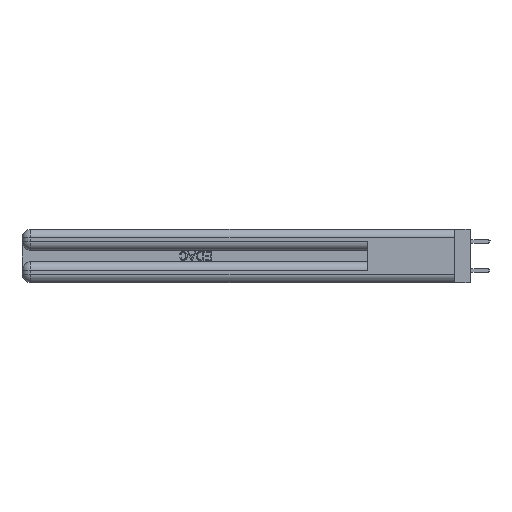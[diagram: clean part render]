
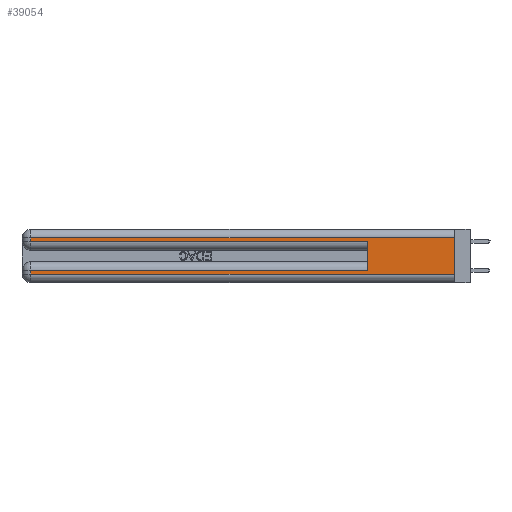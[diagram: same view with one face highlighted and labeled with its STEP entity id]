
A CAD part, left-side view. The second image highlights one B-rep face of the part: STEP entity #39054.
In plain terms, the highlighted planar face has unit normal (-1, 0, 0).
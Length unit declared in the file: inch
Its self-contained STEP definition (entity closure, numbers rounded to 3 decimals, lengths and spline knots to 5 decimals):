
#481 = EDGE_LOOP ( 'NONE', ( #45113, #39682, #36424, #28105, #32733, #26365, #26981, #19928 ) ) ;
#1078 = CARTESIAN_POINT ( 'NONE',  ( 0., 0.6, 0.145 ) ) ;
#2866 = DIRECTION ( 'NONE',  ( 0., 0., -1. ) ) ;
#3239 = CARTESIAN_POINT ( 'NONE',  ( 0., 0.6, 0.085 ) ) ;
#3353 = DIRECTION ( 'NONE',  ( 0., 1., 0. ) ) ;
#3732 = VERTEX_POINT ( 'NONE', #3239 ) ;
#5696 = DIRECTION ( 'NONE',  ( 1., 0., 0. ) ) ;
#6224 = VECTOR ( 'NONE', #2866, 39.37008 ) ;
#7270 = CARTESIAN_POINT ( 'NONE',  ( 0., 0., 0.285 ) ) ;
#7310 = DIRECTION ( 'NONE',  ( 0., 1., 0. ) ) ;
#7464 = LINE ( 'NONE', #50279, #6224 ) ;
#8443 = FACE_OUTER_BOUND ( 'NONE', #481, .T. ) ;
#10803 = LINE ( 'NONE', #7270, #39907 ) ;
#11303 = DIRECTION ( 'NONE',  ( 0., -1., 0. ) ) ;
#11485 = VERTEX_POINT ( 'NONE', #17753 ) ;
#12801 = CARTESIAN_POINT ( 'NONE',  ( 0., 0.6, 0.285 ) ) ;
#16050 = EDGE_CURVE ( 'NONE', #3732, #44000, #24509, .T. ) ;
#16566 = CARTESIAN_POINT ( 'NONE',  ( 0., 2.94, 0.085 ) ) ;
#17489 = VECTOR ( 'NONE', #24978, 39.37008 ) ;
#17753 = CARTESIAN_POINT ( 'NONE',  ( 0., 2.94, 0.06 ) ) ;
#18717 = LINE ( 'NONE', #1078, #17489 ) ;
#19928 = ORIENTED_EDGE ( 'NONE', *, *, #29852, .T. ) ;
#20845 = LINE ( 'NONE', #24901, #50983 ) ;
#24063 = EDGE_CURVE ( 'NONE', #33471, #24924, #10803, .T. ) ;
#24100 = AXIS2_PLACEMENT_3D ( 'NONE', #33316, #5696, #33477 ) ;
#24509 = LINE ( 'NONE', #42962, #33781 ) ;
#24901 = CARTESIAN_POINT ( 'NONE',  ( 0., 2.94, 0.37 ) ) ;
#24924 = VERTEX_POINT ( 'NONE', #12801 ) ;
#24978 = DIRECTION ( 'NONE',  ( 0., 0., 1. ) ) ;
#26365 = ORIENTED_EDGE ( 'NONE', *, *, #16050, .T. ) ;
#26981 = ORIENTED_EDGE ( 'NONE', *, *, #51088, .T. ) ;
#27733 = VECTOR ( 'NONE', #3353, 39.37008 ) ;
#28105 = ORIENTED_EDGE ( 'NONE', *, *, #24063, .T. ) ;
#28912 = DIRECTION ( 'NONE',  ( 0., 0., -1. ) ) ;
#29246 = VECTOR ( 'NONE', #35326, 39.37008 ) ;
#29548 = PLANE ( 'NONE',  #24100 ) ;
#29852 = EDGE_CURVE ( 'NONE', #11485, #31532, #30468, .T. ) ;
#30468 = LINE ( 'NONE', #31371, #29246 ) ;
#31371 = CARTESIAN_POINT ( 'NONE',  ( 0., 0., 0.06 ) ) ;
#31532 = VERTEX_POINT ( 'NONE', #33469 ) ;
#32722 = EDGE_CURVE ( 'NONE', #33329, #31532, #34468, .T. ) ;
#32733 = ORIENTED_EDGE ( 'NONE', *, *, #42719, .F. ) ;
#33246 = VECTOR ( 'NONE', #37517, 39.37008 ) ;
#33316 = CARTESIAN_POINT ( 'NONE',  ( 0., 0., 0.37 ) ) ;
#33329 = VERTEX_POINT ( 'NONE', #40905 ) ;
#33469 = CARTESIAN_POINT ( 'NONE',  ( 0., 0., 0.06 ) ) ;
#33471 = VERTEX_POINT ( 'NONE', #37632 ) ;
#33477 = DIRECTION ( 'NONE',  ( 0., 0., -1. ) ) ;
#33537 = CARTESIAN_POINT ( 'NONE',  ( 0., 0., 0.37 ) ) ;
#33781 = VECTOR ( 'NONE', #7310, 39.37008 ) ;
#34468 = LINE ( 'NONE', #33537, #33246 ) ;
#35326 = DIRECTION ( 'NONE',  ( 0., -1., 0. ) ) ;
#36424 = ORIENTED_EDGE ( 'NONE', *, *, #40187, .T. ) ;
#36935 = VERTEX_POINT ( 'NONE', #50086 ) ;
#37517 = DIRECTION ( 'NONE',  ( 0., 0., -1. ) ) ;
#37632 = CARTESIAN_POINT ( 'NONE',  ( 0., 2.94, 0.285 ) ) ;
#39054 = ADVANCED_FACE ( 'NONE', ( #8443 ), #29548, .F. ) ;
#39423 = LINE ( 'NONE', #50756, #27733 ) ;
#39682 = ORIENTED_EDGE ( 'NONE', *, *, #48251, .T. ) ;
#39907 = VECTOR ( 'NONE', #11303, 39.37008 ) ;
#40187 = EDGE_CURVE ( 'NONE', #36935, #33471, #20845, .T. ) ;
#40905 = CARTESIAN_POINT ( 'NONE',  ( 0., 0., 0.31 ) ) ;
#42719 = EDGE_CURVE ( 'NONE', #3732, #24924, #18717, .T. ) ;
#42962 = CARTESIAN_POINT ( 'NONE',  ( 0., 0., 0.085 ) ) ;
#44000 = VERTEX_POINT ( 'NONE', #16566 ) ;
#45113 = ORIENTED_EDGE ( 'NONE', *, *, #32722, .F. ) ;
#48251 = EDGE_CURVE ( 'NONE', #33329, #36935, #39423, .T. ) ;
#50086 = CARTESIAN_POINT ( 'NONE',  ( 0., 2.94, 0.31 ) ) ;
#50279 = CARTESIAN_POINT ( 'NONE',  ( 0., 2.94, 0.37 ) ) ;
#50756 = CARTESIAN_POINT ( 'NONE',  ( 0., 0., 0.31 ) ) ;
#50983 = VECTOR ( 'NONE', #28912, 39.37008 ) ;
#51088 = EDGE_CURVE ( 'NONE', #44000, #11485, #7464, .T. ) ;
